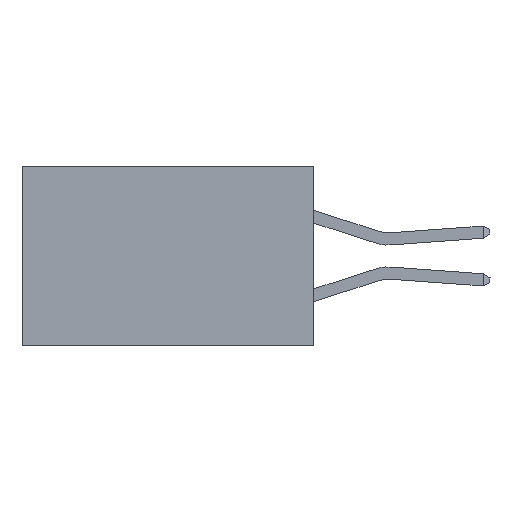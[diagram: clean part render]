
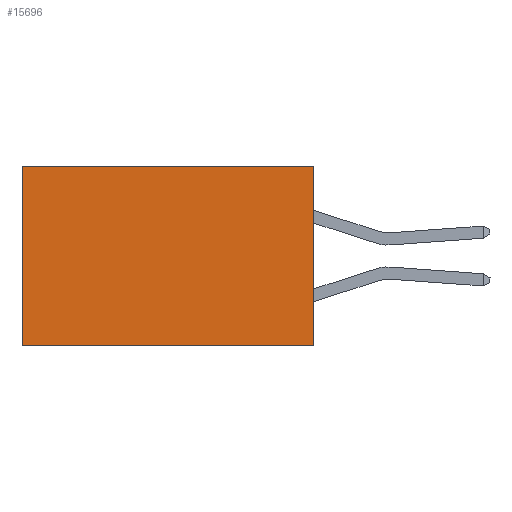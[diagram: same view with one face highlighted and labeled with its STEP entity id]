
A CAD part, left-side view. The second image highlights one B-rep face of the part: STEP entity #15696.
In plain terms, the highlighted planar face has unit normal (-1, 0, 0).
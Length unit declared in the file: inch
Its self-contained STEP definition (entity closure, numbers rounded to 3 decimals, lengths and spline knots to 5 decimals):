
#228 = DIRECTION ( 'NONE',  ( 0., 0., -1. ) ) ;
#233 = ORIENTED_EDGE ( 'NONE', *, *, #7284, .F. ) ;
#640 = EDGE_CURVE ( 'NONE', #4416, #14097, #13869, .T. ) ;
#2171 = CARTESIAN_POINT ( 'NONE',  ( 0.2875, 0., 0. ) ) ;
#2254 = CARTESIAN_POINT ( 'NONE',  ( 0.2875, 0., -0.37 ) ) ;
#2451 = CARTESIAN_POINT ( 'NONE',  ( 0.2875, 0., -0.37 ) ) ;
#3272 = LINE ( 'NONE', #9811, #10547 ) ;
#3424 = VECTOR ( 'NONE', #16010, 39.37008 ) ;
#3591 = DIRECTION ( 'NONE',  ( 0., 1., 0. ) ) ;
#4416 = VERTEX_POINT ( 'NONE', #2451 ) ;
#4719 = VECTOR ( 'NONE', #3591, 39.37008 ) ;
#5773 = ORIENTED_EDGE ( 'NONE', *, *, #15174, .T. ) ;
#6559 = AXIS2_PLACEMENT_3D ( 'NONE', #7436, #16818, #8759 ) ;
#6640 = EDGE_LOOP ( 'NONE', ( #12018, #13847, #233, #5773 ) ) ;
#6821 = CARTESIAN_POINT ( 'NONE',  ( 0.2875, 0., 0. ) ) ;
#7110 = DIRECTION ( 'NONE',  ( 0., 0., -1. ) ) ;
#7284 = EDGE_CURVE ( 'NONE', #8952, #4416, #3272, .T. ) ;
#7436 = CARTESIAN_POINT ( 'NONE',  ( 0.2875, 0., 0. ) ) ;
#8236 = CARTESIAN_POINT ( 'NONE',  ( 0.2875, 0.6, -0.37 ) ) ;
#8759 = DIRECTION ( 'NONE',  ( 0., 0., -1. ) ) ;
#8952 = VERTEX_POINT ( 'NONE', #6821 ) ;
#9811 = CARTESIAN_POINT ( 'NONE',  ( 0.2875, 0., 0. ) ) ;
#10547 = VECTOR ( 'NONE', #7110, 39.37008 ) ;
#10638 = FACE_OUTER_BOUND ( 'NONE', #6640, .T. ) ;
#11156 = VERTEX_POINT ( 'NONE', #11896 ) ;
#11896 = CARTESIAN_POINT ( 'NONE',  ( 0.2875, 0.6, 0. ) ) ;
#12018 = ORIENTED_EDGE ( 'NONE', *, *, #13661, .T. ) ;
#12635 = VECTOR ( 'NONE', #228, 39.37008 ) ;
#13069 = LINE ( 'NONE', #16706, #12635 ) ;
#13661 = EDGE_CURVE ( 'NONE', #11156, #14097, #13069, .T. ) ;
#13847 = ORIENTED_EDGE ( 'NONE', *, *, #640, .F. ) ;
#13869 = LINE ( 'NONE', #2254, #3424 ) ;
#14097 = VERTEX_POINT ( 'NONE', #8236 ) ;
#15174 = EDGE_CURVE ( 'NONE', #8952, #11156, #15487, .T. ) ;
#15480 = PLANE ( 'NONE',  #6559 ) ;
#15487 = LINE ( 'NONE', #2171, #4719 ) ;
#15696 = ADVANCED_FACE ( 'NONE', ( #10638 ), #15480, .F. ) ;
#16010 = DIRECTION ( 'NONE',  ( 0., 1., 0. ) ) ;
#16706 = CARTESIAN_POINT ( 'NONE',  ( 0.2875, 0.6, 0. ) ) ;
#16818 = DIRECTION ( 'NONE',  ( 1., 0., 0. ) ) ;
